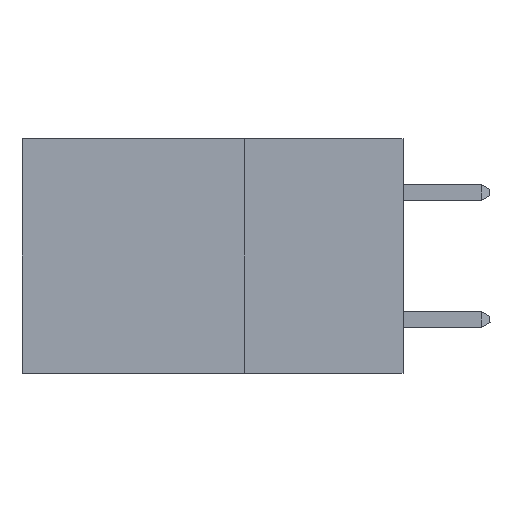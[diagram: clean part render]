
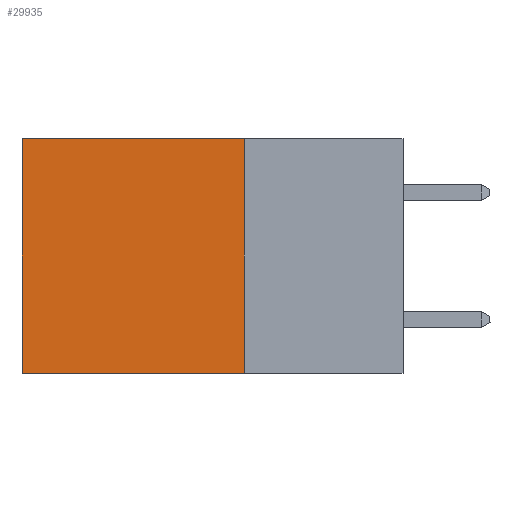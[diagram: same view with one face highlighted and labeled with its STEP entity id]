
A CAD part, left-side view. The second image highlights one B-rep face of the part: STEP entity #29935.
In plain terms, the highlighted planar face has unit normal (-1, 0, 0).
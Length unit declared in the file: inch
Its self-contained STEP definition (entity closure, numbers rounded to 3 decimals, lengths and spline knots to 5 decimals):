
#30 = VERTEX_POINT ( 'NONE', #20233 ) ;
#308 = DIRECTION ( 'NONE',  ( 0., 1., 0. ) ) ;
#766 = CARTESIAN_POINT ( 'NONE',  ( 0.2875, 0.25, 0. ) ) ;
#2157 = EDGE_LOOP ( 'NONE', ( #32824, #24913, #4447, #30789 ) ) ;
#3022 = CARTESIAN_POINT ( 'NONE',  ( 0.2875, 0.6, 0. ) ) ;
#4447 = ORIENTED_EDGE ( 'NONE', *, *, #5586, .F. ) ;
#4852 = DIRECTION ( 'NONE',  ( 1., 0., 0. ) ) ;
#5586 = EDGE_CURVE ( 'NONE', #25000, #15731, #17123, .T. ) ;
#7720 = LINE ( 'NONE', #8024, #8510 ) ;
#7971 = CARTESIAN_POINT ( 'NONE',  ( 0.2875, 0.25, -0.37 ) ) ;
#8024 = CARTESIAN_POINT ( 'NONE',  ( 0.2875, 0.6, 0. ) ) ;
#8510 = VECTOR ( 'NONE', #23807, 39.37008 ) ;
#9342 = LINE ( 'NONE', #766, #13411 ) ;
#10206 = VECTOR ( 'NONE', #21803, 39.37008 ) ;
#10259 = FACE_OUTER_BOUND ( 'NONE', #2157, .T. ) ;
#12987 = DIRECTION ( 'NONE',  ( 0., 1., 0. ) ) ;
#13411 = VECTOR ( 'NONE', #308, 39.37008 ) ;
#13602 = AXIS2_PLACEMENT_3D ( 'NONE', #27782, #4852, #28113 ) ;
#15153 = EDGE_CURVE ( 'NONE', #23469, #30, #7720, .T. ) ;
#15731 = VERTEX_POINT ( 'NONE', #26716 ) ;
#16220 = CARTESIAN_POINT ( 'NONE',  ( 0.2875, 0.25, 0. ) ) ;
#17123 = LINE ( 'NONE', #24280, #10206 ) ;
#17787 = PLANE ( 'NONE',  #13602 ) ;
#20233 = CARTESIAN_POINT ( 'NONE',  ( 0.2875, 0.6, -0.37 ) ) ;
#21803 = DIRECTION ( 'NONE',  ( 0., 0., -1. ) ) ;
#23469 = VERTEX_POINT ( 'NONE', #3022 ) ;
#23807 = DIRECTION ( 'NONE',  ( 0., 0., -1. ) ) ;
#24280 = CARTESIAN_POINT ( 'NONE',  ( 0.2875, 0.25, 0. ) ) ;
#24667 = LINE ( 'NONE', #7971, #28726 ) ;
#24913 = ORIENTED_EDGE ( 'NONE', *, *, #26984, .F. ) ;
#24981 = EDGE_CURVE ( 'NONE', #25000, #23469, #9342, .T. ) ;
#25000 = VERTEX_POINT ( 'NONE', #16220 ) ;
#26716 = CARTESIAN_POINT ( 'NONE',  ( 0.2875, 0.25, -0.37 ) ) ;
#26984 = EDGE_CURVE ( 'NONE', #15731, #30, #24667, .T. ) ;
#27782 = CARTESIAN_POINT ( 'NONE',  ( 0.2875, 0.25, 0. ) ) ;
#28113 = DIRECTION ( 'NONE',  ( 0., 0., -1. ) ) ;
#28726 = VECTOR ( 'NONE', #12987, 39.37008 ) ;
#29935 = ADVANCED_FACE ( 'NONE', ( #10259 ), #17787, .F. ) ;
#30789 = ORIENTED_EDGE ( 'NONE', *, *, #24981, .T. ) ;
#32824 = ORIENTED_EDGE ( 'NONE', *, *, #15153, .T. ) ;
